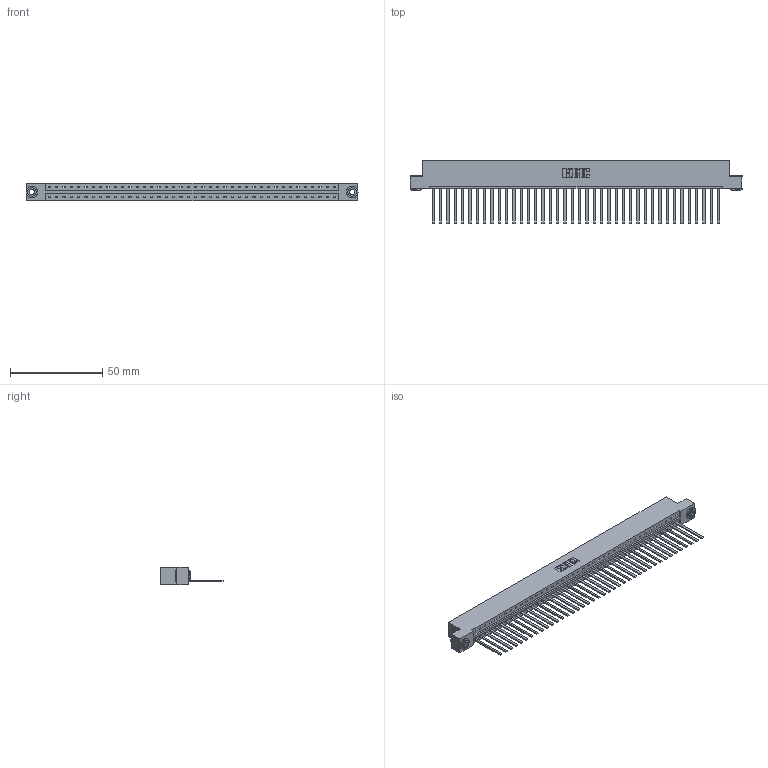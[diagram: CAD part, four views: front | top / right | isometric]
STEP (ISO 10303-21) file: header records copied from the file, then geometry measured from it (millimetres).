
FILE_DESCRIPTION (( 'STEP AP203' ), '1' );
FILE_NAME ('833-040-544-103.STEP', '2020-06-03T17:25:01', ( '' ), ( '' ), 'SwSTEP 2.0', 'SolidWorks 2020', '' );
FILE_SCHEMA (( 'CONFIG_CONTROL_DESIGN' ));
Length unit declared in the file: inch
Products named in the file (4): 833-040-544-103; 345-292-001_345-293-144; 833 Part_Flush - .156 Dia - TH; 345-250-002_345-250-002-102
Assembly tree (43 placements, depth 2):
  833-040-544-103
    833 Part_Flush - .156 Dia - TH
    345-292-001_345-293-144  x40
    345-250-002_345-250-002-102  x2
Bounding box: 180.04 x 34.3 x 9.4 mm (x, y, z)
Volume: 18582.1 mm3; surface area: 21826.3 mm2
Topology: 43 solids, 43 shells, 2232 faces, 6707 edges, 4414 vertices
Faces by surface type: plane 1600, cylinder 624, cone 8
Entity records: 25178 total; most frequent: CARTESIAN_POINT 4321, ORIENTED_EDGE 4290, DIRECTION 3679, EDGE_CURVE 2145, VECTOR 1997, LINE 1997, VERTEX_POINT 1426, AXIS2_PLACEMENT_3D 841
